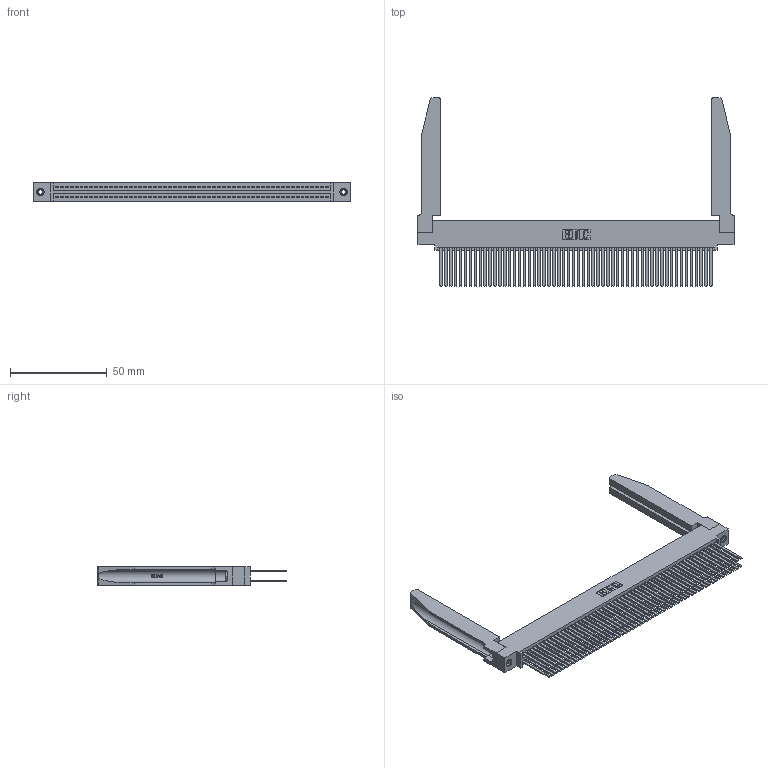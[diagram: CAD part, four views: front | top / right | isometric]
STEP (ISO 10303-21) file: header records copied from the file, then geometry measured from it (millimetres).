
FILE_DESCRIPTION (( 'STEP AP203' ), '1' );
FILE_NAME ('345-112-544-578.STEP', '2019-11-04T22:29:15', ( '' ), ( '' ), 'SwSTEP 2.0', 'SolidWorks 2016', '' );
FILE_SCHEMA (( 'CONFIG_CONTROL_DESIGN' ));
Length unit declared in the file: inch
Products named in the file (5): 345-250-001_345-250-001-102; 345 Part_0.110 Offset - 0.156 Dia-TH; 345-292-001_345-293-144; 345-112-544-578; 345-220-078_345-220-078
Assembly tree (117 placements, depth 2):
  345-112-544-578
    345 Part_0.110 Offset - 0.156 Dia-TH
    345-292-001_345-293-144  x112
    345-250-001_345-250-001-102  x2
    345-220-078_345-220-078  x2
Bounding box: 163.47 x 97.71 x 9.4 mm (x, y, z)
Volume: 25277.1 mm3; surface area: 37681.9 mm2
Topology: 117 solids, 117 shells, 5292 faces, 15633 edges, 10262 vertices
Faces by surface type: plane 3474, cylinder 1766, bspline 36, cone 12, torus 4
Entity records: 46742 total; most frequent: CARTESIAN_POINT 8739, ORIENTED_EDGE 7570, DIRECTION 6679, EDGE_CURVE 3785, LINE 3339, VECTOR 3339, VERTEX_POINT 2516, AXIS2_PLACEMENT_3D 1670
